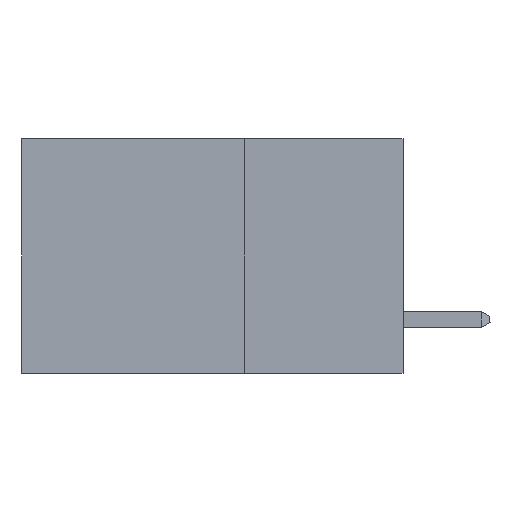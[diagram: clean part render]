
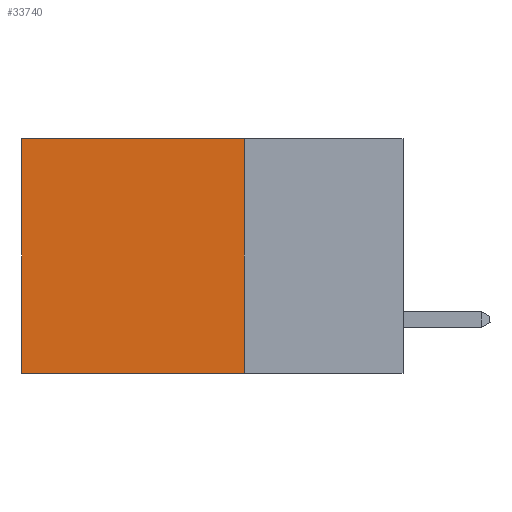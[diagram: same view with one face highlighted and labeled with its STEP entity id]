
A CAD part, left-side view. The second image highlights one B-rep face of the part: STEP entity #33740.
In plain terms, the highlighted planar face has unit normal (-1, 0, 0).
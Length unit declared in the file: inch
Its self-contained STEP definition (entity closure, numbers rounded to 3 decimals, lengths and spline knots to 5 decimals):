
#1517 = LINE ( 'NONE', #44543, #28137 ) ;
#3317 = CARTESIAN_POINT ( 'NONE',  ( 0.2875, 0.6, 0. ) ) ;
#5353 = ORIENTED_EDGE ( 'NONE', *, *, #15510, .F. ) ;
#6232 = CARTESIAN_POINT ( 'NONE',  ( 0.2875, 0.25, 0. ) ) ;
#11606 = CARTESIAN_POINT ( 'NONE',  ( 0.2875, 0.25, 0. ) ) ;
#11718 = VECTOR ( 'NONE', #15171, 39.37008 ) ;
#15152 = CARTESIAN_POINT ( 'NONE',  ( 0.2875, 0.25, -0.37 ) ) ;
#15171 = DIRECTION ( 'NONE',  ( 0., 1., 0. ) ) ;
#15510 = EDGE_CURVE ( 'NONE', #29731, #44582, #38561, .T. ) ;
#16222 = CARTESIAN_POINT ( 'NONE',  ( 0.2875, 0.25, -0.37 ) ) ;
#16732 = EDGE_CURVE ( 'NONE', #29731, #41111, #50179, .T. ) ;
#17720 = VERTEX_POINT ( 'NONE', #38401 ) ;
#17923 = ORIENTED_EDGE ( 'NONE', *, *, #16732, .T. ) ;
#22692 = ORIENTED_EDGE ( 'NONE', *, *, #23195, .T. ) ;
#23195 = EDGE_CURVE ( 'NONE', #41111, #17720, #1517, .T. ) ;
#23879 = DIRECTION ( 'NONE',  ( 0., 0., -1. ) ) ;
#24042 = DIRECTION ( 'NONE',  ( 0., 1., 0. ) ) ;
#24441 = VECTOR ( 'NONE', #24042, 39.37008 ) ;
#26007 = DIRECTION ( 'NONE',  ( 0., 0., -1. ) ) ;
#27294 = FACE_OUTER_BOUND ( 'NONE', #39214, .T. ) ;
#28137 = VECTOR ( 'NONE', #26007, 39.37008 ) ;
#29731 = VERTEX_POINT ( 'NONE', #6232 ) ;
#32148 = CARTESIAN_POINT ( 'NONE',  ( 0.2875, 0.25, 0. ) ) ;
#33075 = ORIENTED_EDGE ( 'NONE', *, *, #48771, .F. ) ;
#33740 = ADVANCED_FACE ( 'NONE', ( #27294 ), #39954, .F. ) ;
#35438 = CARTESIAN_POINT ( 'NONE',  ( 0.2875, 0.25, 0. ) ) ;
#35796 = DIRECTION ( 'NONE',  ( 1., 0., 0. ) ) ;
#36189 = LINE ( 'NONE', #16222, #24441 ) ;
#38401 = CARTESIAN_POINT ( 'NONE',  ( 0.2875, 0.6, -0.37 ) ) ;
#38561 = LINE ( 'NONE', #11606, #46026 ) ;
#39214 = EDGE_LOOP ( 'NONE', ( #22692, #33075, #5353, #17923 ) ) ;
#39954 = PLANE ( 'NONE',  #47412 ) ;
#41111 = VERTEX_POINT ( 'NONE', #3317 ) ;
#43687 = DIRECTION ( 'NONE',  ( 0., 0., -1. ) ) ;
#44543 = CARTESIAN_POINT ( 'NONE',  ( 0.2875, 0.6, 0. ) ) ;
#44582 = VERTEX_POINT ( 'NONE', #15152 ) ;
#46026 = VECTOR ( 'NONE', #43687, 39.37008 ) ;
#47412 = AXIS2_PLACEMENT_3D ( 'NONE', #32148, #35796, #23879 ) ;
#48771 = EDGE_CURVE ( 'NONE', #44582, #17720, #36189, .T. ) ;
#50179 = LINE ( 'NONE', #35438, #11718 ) ;
